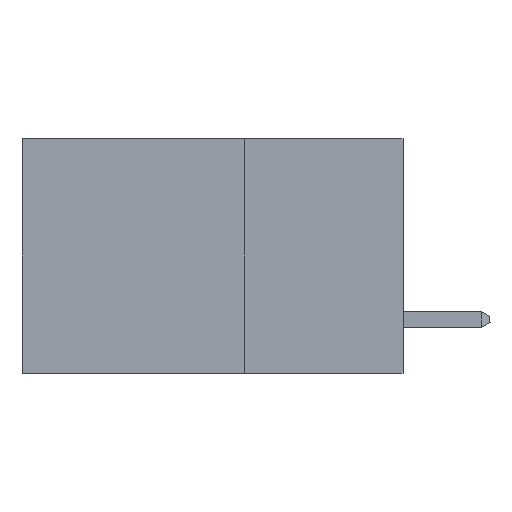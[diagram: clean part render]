
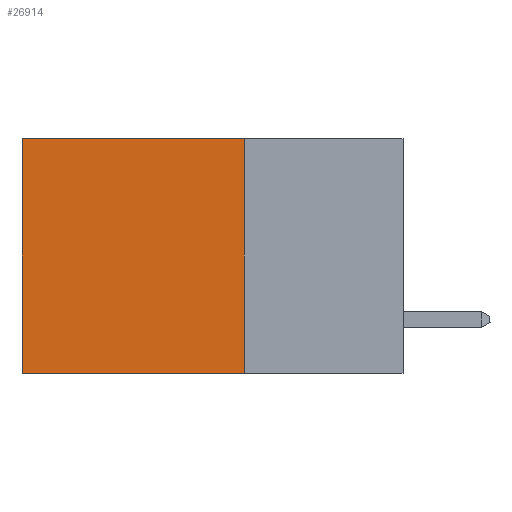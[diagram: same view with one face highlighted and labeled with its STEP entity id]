
A CAD part, left-side view. The second image highlights one B-rep face of the part: STEP entity #26914.
In plain terms, the highlighted planar face has unit normal (-1, 0, 0).
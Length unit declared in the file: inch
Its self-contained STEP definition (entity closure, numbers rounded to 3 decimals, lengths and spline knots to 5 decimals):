
#95 = VECTOR ( 'NONE', #27986, 39.37008 ) ;
#1092 = VERTEX_POINT ( 'NONE', #2723 ) ;
#1327 = CARTESIAN_POINT ( 'NONE',  ( 0.2875, 0.25, 0. ) ) ;
#1815 = EDGE_CURVE ( 'NONE', #17975, #15975, #27664, .T. ) ;
#1900 = VECTOR ( 'NONE', #22482, 39.37008 ) ;
#2723 = CARTESIAN_POINT ( 'NONE',  ( 0.2875, 0.25, 0. ) ) ;
#3059 = ORIENTED_EDGE ( 'NONE', *, *, #15881, .F. ) ;
#4221 = DIRECTION ( 'NONE',  ( 0., 1., 0. ) ) ;
#4916 = VERTEX_POINT ( 'NONE', #33096 ) ;
#6539 = CARTESIAN_POINT ( 'NONE',  ( 0.2875, 0.25, -0.37 ) ) ;
#7064 = CARTESIAN_POINT ( 'NONE',  ( 0.2875, 0.6, -0.37 ) ) ;
#7544 = PLANE ( 'NONE',  #23983 ) ;
#9611 = LINE ( 'NONE', #6539, #26451 ) ;
#12059 = CARTESIAN_POINT ( 'NONE',  ( 0.2875, 0.25, 0. ) ) ;
#12376 = CARTESIAN_POINT ( 'NONE',  ( 0.2875, 0.6, 0. ) ) ;
#12954 = VECTOR ( 'NONE', #4221, 39.37008 ) ;
#15881 = EDGE_CURVE ( 'NONE', #4916, #15975, #9611, .T. ) ;
#15974 = EDGE_CURVE ( 'NONE', #1092, #17975, #16970, .T. ) ;
#15975 = VERTEX_POINT ( 'NONE', #7064 ) ;
#16970 = LINE ( 'NONE', #12059, #12954 ) ;
#17130 = LINE ( 'NONE', #1327, #1900 ) ;
#17203 = DIRECTION ( 'NONE',  ( 0., 1., 0. ) ) ;
#17975 = VERTEX_POINT ( 'NONE', #30388 ) ;
#20527 = DIRECTION ( 'NONE',  ( 0., 0., -1. ) ) ;
#20767 = DIRECTION ( 'NONE',  ( 1., 0., 0. ) ) ;
#21572 = EDGE_LOOP ( 'NONE', ( #32064, #3059, #31402, #31420 ) ) ;
#22482 = DIRECTION ( 'NONE',  ( 0., 0., -1. ) ) ;
#23153 = FACE_OUTER_BOUND ( 'NONE', #21572, .T. ) ;
#23983 = AXIS2_PLACEMENT_3D ( 'NONE', #28821, #20767, #20527 ) ;
#26451 = VECTOR ( 'NONE', #17203, 39.37008 ) ;
#26914 = ADVANCED_FACE ( 'NONE', ( #23153 ), #7544, .F. ) ;
#27664 = LINE ( 'NONE', #12376, #95 ) ;
#27986 = DIRECTION ( 'NONE',  ( 0., 0., -1. ) ) ;
#28821 = CARTESIAN_POINT ( 'NONE',  ( 0.2875, 0.25, 0. ) ) ;
#30388 = CARTESIAN_POINT ( 'NONE',  ( 0.2875, 0.6, 0. ) ) ;
#31402 = ORIENTED_EDGE ( 'NONE', *, *, #32977, .F. ) ;
#31420 = ORIENTED_EDGE ( 'NONE', *, *, #15974, .T. ) ;
#32064 = ORIENTED_EDGE ( 'NONE', *, *, #1815, .T. ) ;
#32977 = EDGE_CURVE ( 'NONE', #1092, #4916, #17130, .T. ) ;
#33096 = CARTESIAN_POINT ( 'NONE',  ( 0.2875, 0.25, -0.37 ) ) ;
